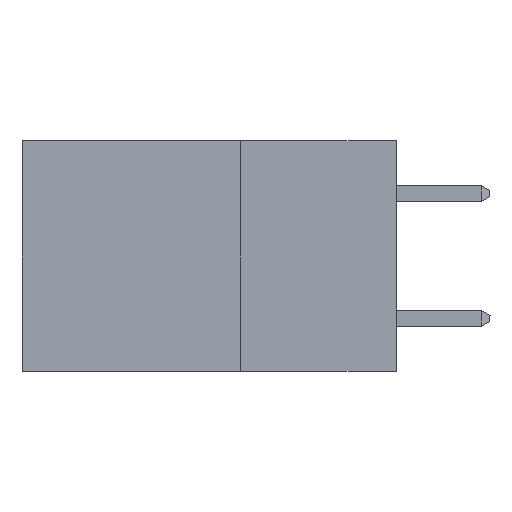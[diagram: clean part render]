
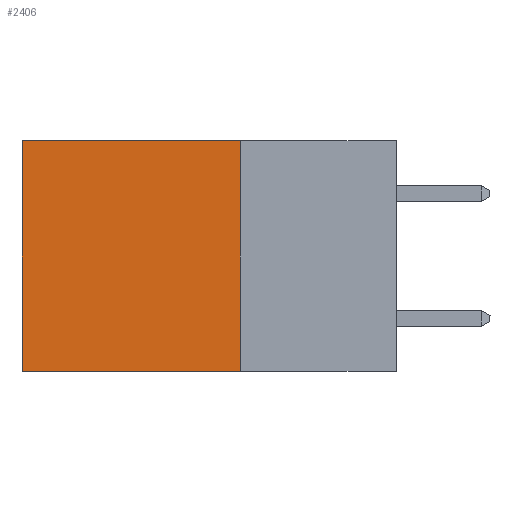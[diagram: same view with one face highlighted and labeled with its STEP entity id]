
A CAD part, left-side view. The second image highlights one B-rep face of the part: STEP entity #2406.
In plain terms, the highlighted planar face has unit normal (-1, 0, 0).
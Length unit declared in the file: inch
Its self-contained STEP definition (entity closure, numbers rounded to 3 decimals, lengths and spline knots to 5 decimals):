
#617 = VERTEX_POINT ( 'NONE', #8678 ) ;
#749 = CARTESIAN_POINT ( 'NONE',  ( 0.2615, 0.25, -0.37 ) ) ;
#2406 = ADVANCED_FACE ( 'NONE', ( #9576 ), #8755, .F. ) ;
#2442 = DIRECTION ( 'NONE',  ( 0., 0., -1. ) ) ;
#2444 = AXIS2_PLACEMENT_3D ( 'NONE', #749, #11847, #2442 ) ;
#2570 = VECTOR ( 'NONE', #5045, 39.37008 ) ;
#2907 = CARTESIAN_POINT ( 'NONE',  ( 0.2615, 0.25, 0. ) ) ;
#3065 = LINE ( 'NONE', #9807, #2570 ) ;
#3123 = EDGE_CURVE ( 'NONE', #9446, #617, #15419, .T. ) ;
#4621 = CARTESIAN_POINT ( 'NONE',  ( 0.2615, 0.25, -0.37 ) ) ;
#5045 = DIRECTION ( 'NONE',  ( 0., 1., 0. ) ) ;
#5342 = EDGE_CURVE ( 'NONE', #11826, #9446, #14475, .T. ) ;
#7365 = ORIENTED_EDGE ( 'NONE', *, *, #3123, .F. ) ;
#7601 = EDGE_CURVE ( 'NONE', #9953, #617, #12427, .T. ) ;
#8332 = VECTOR ( 'NONE', #12873, 39.37008 ) ;
#8678 = CARTESIAN_POINT ( 'NONE',  ( 0.2615, 0.6, -0.37 ) ) ;
#8755 = PLANE ( 'NONE',  #2444 ) ;
#9149 = ORIENTED_EDGE ( 'NONE', *, *, #14641, .T. ) ;
#9446 = VERTEX_POINT ( 'NONE', #19430 ) ;
#9576 = FACE_OUTER_BOUND ( 'NONE', #12538, .T. ) ;
#9784 = CARTESIAN_POINT ( 'NONE',  ( 0.2615, 0.6, -0.37 ) ) ;
#9807 = CARTESIAN_POINT ( 'NONE',  ( 0.2615, 0.25, 0. ) ) ;
#9953 = VERTEX_POINT ( 'NONE', #17520 ) ;
#9962 = VECTOR ( 'NONE', #15389, 39.37008 ) ;
#11826 = VERTEX_POINT ( 'NONE', #2907 ) ;
#11847 = DIRECTION ( 'NONE',  ( 1., 0., 0. ) ) ;
#12427 = LINE ( 'NONE', #9784, #8332 ) ;
#12538 = EDGE_LOOP ( 'NONE', ( #17427, #7365, #15337, #9149 ) ) ;
#12873 = DIRECTION ( 'NONE',  ( 0., 0., -1. ) ) ;
#14475 = LINE ( 'NONE', #4621, #9962 ) ;
#14641 = EDGE_CURVE ( 'NONE', #11826, #9953, #3065, .T. ) ;
#15337 = ORIENTED_EDGE ( 'NONE', *, *, #5342, .F. ) ;
#15389 = DIRECTION ( 'NONE',  ( 0., 0., -1. ) ) ;
#15419 = LINE ( 'NONE', #17845, #18895 ) ;
#17427 = ORIENTED_EDGE ( 'NONE', *, *, #7601, .T. ) ;
#17520 = CARTESIAN_POINT ( 'NONE',  ( 0.2615, 0.6, 0. ) ) ;
#17845 = CARTESIAN_POINT ( 'NONE',  ( 0.2615, 0.25, -0.37 ) ) ;
#18895 = VECTOR ( 'NONE', #19358, 39.37008 ) ;
#19358 = DIRECTION ( 'NONE',  ( 0., 1., 0. ) ) ;
#19430 = CARTESIAN_POINT ( 'NONE',  ( 0.2615, 0.25, -0.37 ) ) ;
